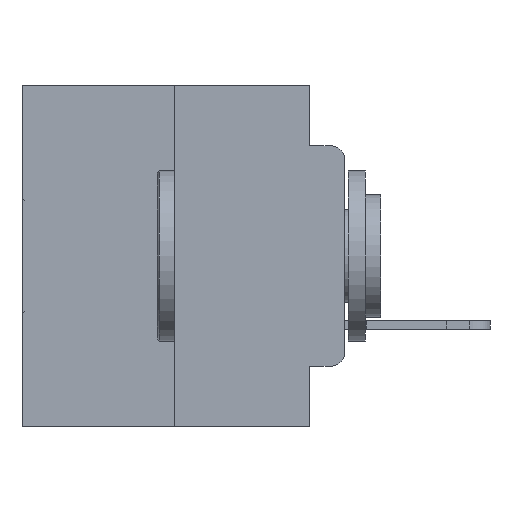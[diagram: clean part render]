
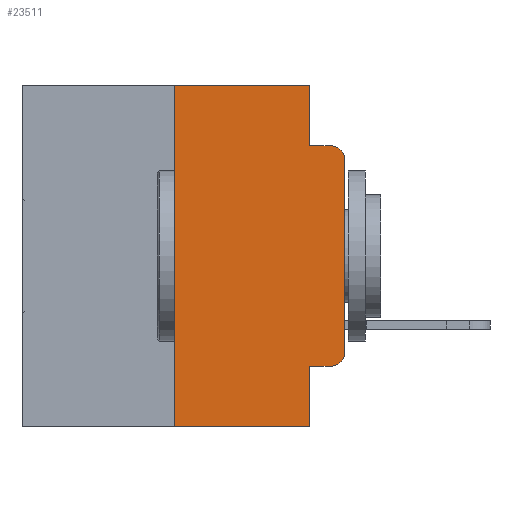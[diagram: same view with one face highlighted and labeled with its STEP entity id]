
A CAD part, left-side view. The second image highlights one B-rep face of the part: STEP entity #23511.
In plain terms, the highlighted planar face has unit normal (-1, 0, 0).
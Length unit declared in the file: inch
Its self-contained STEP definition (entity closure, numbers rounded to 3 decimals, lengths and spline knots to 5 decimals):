
#426 = VECTOR ( 'NONE', #5558, 39.37008 ) ;
#436 = CARTESIAN_POINT ( 'NONE',  ( 0., 0.02, -0.0885 ) ) ;
#575 = VERTEX_POINT ( 'NONE', #29585 ) ;
#1268 = LINE ( 'NONE', #9264, #20421 ) ;
#1779 = VERTEX_POINT ( 'NONE', #29039 ) ;
#2078 = DIRECTION ( 'NONE',  ( 0., 0., -1. ) ) ;
#2350 = VERTEX_POINT ( 'NONE', #13242 ) ;
#2611 = CARTESIAN_POINT ( 'NONE',  ( 0., 0., -0.1085 ) ) ;
#2629 = VERTEX_POINT ( 'NONE', #12099 ) ;
#3270 = VERTEX_POINT ( 'NONE', #2611 ) ;
#3641 = ORIENTED_EDGE ( 'NONE', *, *, #9207, .F. ) ;
#3823 = CARTESIAN_POINT ( 'NONE',  ( 0., 0.051, -0.0885 ) ) ;
#4056 = FACE_OUTER_BOUND ( 'NONE', #24935, .T. ) ;
#4332 = VERTEX_POINT ( 'NONE', #24497 ) ;
#4374 = EDGE_CURVE ( 'NONE', #2350, #3270, #13323, .T. ) ;
#4448 = DIRECTION ( 'NONE',  ( 0., -1., 0. ) ) ;
#4912 = ORIENTED_EDGE ( 'NONE', *, *, #18495, .F. ) ;
#5520 = CARTESIAN_POINT ( 'NONE',  ( 0., 0.051, -0.4115 ) ) ;
#5558 = DIRECTION ( 'NONE',  ( 0., -1., 0. ) ) ;
#5648 = VECTOR ( 'NONE', #30370, 39.37008 ) ;
#6373 = EDGE_CURVE ( 'NONE', #12786, #19412, #26991, .T. ) ;
#7528 = DIRECTION ( 'NONE',  ( 0., 0., -1. ) ) ;
#9160 = DIRECTION ( 'NONE',  ( 0., 0., 1. ) ) ;
#9207 = EDGE_CURVE ( 'NONE', #1779, #2629, #11645, .T. ) ;
#9264 = CARTESIAN_POINT ( 'NONE',  ( 0., 0.25, 0. ) ) ;
#9381 = ORIENTED_EDGE ( 'NONE', *, *, #29143, .T. ) ;
#10331 = EDGE_CURVE ( 'NONE', #4332, #2350, #16260, .T. ) ;
#11645 = LINE ( 'NONE', #23344, #24178 ) ;
#11977 = DIRECTION ( 'NONE',  ( 0., 0., -1. ) ) ;
#11985 = CARTESIAN_POINT ( 'NONE',  ( 0., 0.051, 0. ) ) ;
#12099 = CARTESIAN_POINT ( 'NONE',  ( 0., 0.051, 0. ) ) ;
#12213 = VERTEX_POINT ( 'NONE', #436 ) ;
#12223 = ORIENTED_EDGE ( 'NONE', *, *, #15310, .F. ) ;
#12595 = CARTESIAN_POINT ( 'NONE',  ( 0., 0.051, 0. ) ) ;
#12786 = VERTEX_POINT ( 'NONE', #21060 ) ;
#13242 = CARTESIAN_POINT ( 'NONE',  ( 0., 0., -0.3915 ) ) ;
#13323 = LINE ( 'NONE', #22498, #5648 ) ;
#13710 = EDGE_CURVE ( 'NONE', #575, #4332, #14194, .T. ) ;
#14194 = LINE ( 'NONE', #5520, #426 ) ;
#14258 = ORIENTED_EDGE ( 'NONE', *, *, #13710, .T. ) ;
#14318 = CIRCLE ( 'NONE', #28975, 0.02 ) ;
#15310 = EDGE_CURVE ( 'NONE', #575, #19412, #29406, .T. ) ;
#15330 = CARTESIAN_POINT ( 'NONE',  ( 0., 0.051, -0.0885 ) ) ;
#15675 = ORIENTED_EDGE ( 'NONE', *, *, #20000, .F. ) ;
#15985 = VECTOR ( 'NONE', #11977, 39.37008 ) ;
#16260 = CIRCLE ( 'NONE', #16797, 0.02 ) ;
#16797 = AXIS2_PLACEMENT_3D ( 'NONE', #17982, #17950, #17942 ) ;
#17304 = DIRECTION ( 'NONE',  ( -1., 0., 0. ) ) ;
#17522 = ORIENTED_EDGE ( 'NONE', *, *, #24585, .F. ) ;
#17942 = DIRECTION ( 'NONE',  ( 0., 0., -1. ) ) ;
#17950 = DIRECTION ( 'NONE',  ( -1., 0., 0. ) ) ;
#17982 = CARTESIAN_POINT ( 'NONE',  ( 0., 0.02, -0.3915 ) ) ;
#18495 = EDGE_CURVE ( 'NONE', #12786, #1779, #1268, .T. ) ;
#19412 = VERTEX_POINT ( 'NONE', #27214 ) ;
#19775 = ORIENTED_EDGE ( 'NONE', *, *, #10331, .T. ) ;
#20000 = EDGE_CURVE ( 'NONE', #2629, #26739, #27489, .T. ) ;
#20293 = VECTOR ( 'NONE', #4448, 39.37008 ) ;
#20421 = VECTOR ( 'NONE', #9160, 39.37008 ) ;
#20873 = VECTOR ( 'NONE', #23667, 39.37008 ) ;
#21060 = CARTESIAN_POINT ( 'NONE',  ( 0., 0.25, -0.5 ) ) ;
#22498 = CARTESIAN_POINT ( 'NONE',  ( 0., 0., 0. ) ) ;
#23171 = ORIENTED_EDGE ( 'NONE', *, *, #4374, .T. ) ;
#23206 = DIRECTION ( 'NONE',  ( 0., -1., 0. ) ) ;
#23253 = DIRECTION ( 'NONE',  ( 0., 0., -1. ) ) ;
#23279 = DIRECTION ( 'NONE',  ( 1., 0., 0. ) ) ;
#23285 = PLANE ( 'NONE',  #30795 ) ;
#23344 = CARTESIAN_POINT ( 'NONE',  ( 0., 0.473, 0. ) ) ;
#23350 = VECTOR ( 'NONE', #7528, 39.37008 ) ;
#23472 = CARTESIAN_POINT ( 'NONE',  ( 0., 0.473, 0. ) ) ;
#23511 = ADVANCED_FACE ( 'NONE', ( #4056 ), #23285, .F. ) ;
#23635 = CARTESIAN_POINT ( 'NONE',  ( 0., 0.473, -0.5 ) ) ;
#23667 = DIRECTION ( 'NONE',  ( 0., -1., 0. ) ) ;
#24178 = VECTOR ( 'NONE', #23206, 39.37008 ) ;
#24497 = CARTESIAN_POINT ( 'NONE',  ( 0., 0.02, -0.4115 ) ) ;
#24585 = EDGE_CURVE ( 'NONE', #26739, #12213, #27101, .T. ) ;
#24935 = EDGE_LOOP ( 'NONE', ( #23171, #9381, #17522, #15675, #3641, #4912, #28599, #12223, #14258, #19775 ) ) ;
#26739 = VERTEX_POINT ( 'NONE', #15330 ) ;
#26991 = LINE ( 'NONE', #23635, #20873 ) ;
#27101 = LINE ( 'NONE', #3823, #20293 ) ;
#27214 = CARTESIAN_POINT ( 'NONE',  ( 0., 0.051, -0.5 ) ) ;
#27489 = LINE ( 'NONE', #11985, #15985 ) ;
#28599 = ORIENTED_EDGE ( 'NONE', *, *, #6373, .T. ) ;
#28975 = AXIS2_PLACEMENT_3D ( 'NONE', #30764, #17304, #2078 ) ;
#29039 = CARTESIAN_POINT ( 'NONE',  ( 0., 0.25, 0. ) ) ;
#29143 = EDGE_CURVE ( 'NONE', #3270, #12213, #14318, .T. ) ;
#29406 = LINE ( 'NONE', #12595, #23350 ) ;
#29585 = CARTESIAN_POINT ( 'NONE',  ( 0., 0.051, -0.4115 ) ) ;
#30370 = DIRECTION ( 'NONE',  ( 0., 0., 1. ) ) ;
#30764 = CARTESIAN_POINT ( 'NONE',  ( 0., 0.02, -0.1085 ) ) ;
#30795 = AXIS2_PLACEMENT_3D ( 'NONE', #23472, #23279, #23253 ) ;
